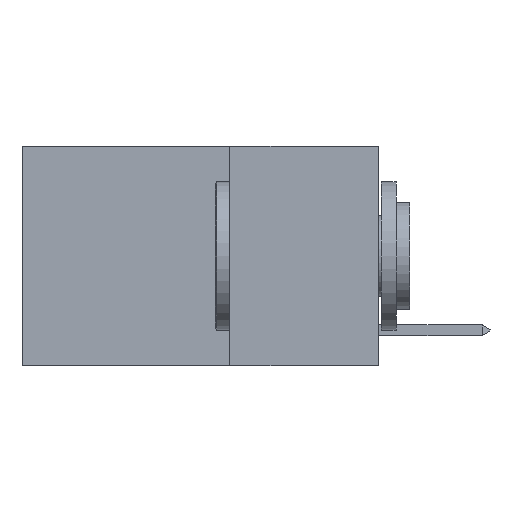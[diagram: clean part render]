
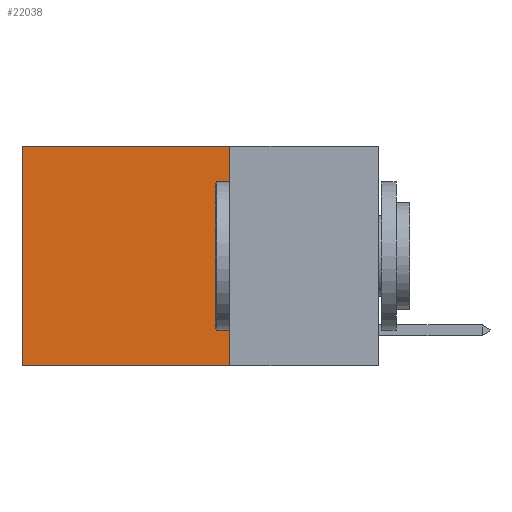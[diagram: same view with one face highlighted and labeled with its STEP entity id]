
A CAD part, left-side view. The second image highlights one B-rep face of the part: STEP entity #22038.
In plain terms, the highlighted planar face has unit normal (-1, 0, 0).
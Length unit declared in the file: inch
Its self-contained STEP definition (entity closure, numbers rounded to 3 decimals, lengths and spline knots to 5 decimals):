
#1754 = ORIENTED_EDGE ( 'NONE', *, *, #24520, .F. ) ;
#2118 = ORIENTED_EDGE ( 'NONE', *, *, #24918, .T. ) ;
#4122 = DIRECTION ( 'NONE',  ( 0., 1., 0. ) ) ;
#4167 = PLANE ( 'NONE',  #25455 ) ;
#5313 = VECTOR ( 'NONE', #19232, 39.37008 ) ;
#6423 = CARTESIAN_POINT ( 'NONE',  ( 0.2625, 0.25, 0. ) ) ;
#6466 = DIRECTION ( 'NONE',  ( 0., 0., -1. ) ) ;
#7605 = EDGE_CURVE ( 'NONE', #13305, #20000, #18055, .T. ) ;
#7867 = CARTESIAN_POINT ( 'NONE',  ( 0.2625, 0.25, -0.37 ) ) ;
#8535 = DIRECTION ( 'NONE',  ( 1., 0., 0. ) ) ;
#10118 = VECTOR ( 'NONE', #4122, 39.37008 ) ;
#10273 = CARTESIAN_POINT ( 'NONE',  ( 0.2625, 0.6, 0. ) ) ;
#10665 = FACE_OUTER_BOUND ( 'NONE', #19498, .T. ) ;
#11126 = ORIENTED_EDGE ( 'NONE', *, *, #19804, .T. ) ;
#12660 = LINE ( 'NONE', #25573, #5313 ) ;
#12701 = CARTESIAN_POINT ( 'NONE',  ( 0.2625, 0.25, 0. ) ) ;
#13259 = CARTESIAN_POINT ( 'NONE',  ( 0.2625, 0.25, 0. ) ) ;
#13305 = VERTEX_POINT ( 'NONE', #7867 ) ;
#14267 = CARTESIAN_POINT ( 'NONE',  ( 0.2625, 0.25, -0.37 ) ) ;
#14719 = ORIENTED_EDGE ( 'NONE', *, *, #7605, .F. ) ;
#14830 = CARTESIAN_POINT ( 'NONE',  ( 0.2625, 0.25, 0. ) ) ;
#15960 = DIRECTION ( 'NONE',  ( 0., 1., 0. ) ) ;
#17042 = LINE ( 'NONE', #12701, #10118 ) ;
#17125 = DIRECTION ( 'NONE',  ( 0., 0., -1. ) ) ;
#18055 = LINE ( 'NONE', #14267, #23469 ) ;
#19232 = DIRECTION ( 'NONE',  ( 0., 0., -1. ) ) ;
#19410 = VERTEX_POINT ( 'NONE', #14830 ) ;
#19498 = EDGE_LOOP ( 'NONE', ( #2118, #14719, #1754, #11126 ) ) ;
#19720 = VECTOR ( 'NONE', #6466, 39.37008 ) ;
#19804 = EDGE_CURVE ( 'NONE', #19410, #20028, #17042, .T. ) ;
#20000 = VERTEX_POINT ( 'NONE', #24901 ) ;
#20028 = VERTEX_POINT ( 'NONE', #10273 ) ;
#22038 = ADVANCED_FACE ( 'NONE', ( #10665 ), #4167, .F. ) ;
#23469 = VECTOR ( 'NONE', #15960, 39.37008 ) ;
#24520 = EDGE_CURVE ( 'NONE', #19410, #13305, #26014, .T. ) ;
#24901 = CARTESIAN_POINT ( 'NONE',  ( 0.2625, 0.6, -0.37 ) ) ;
#24918 = EDGE_CURVE ( 'NONE', #20028, #20000, #12660, .T. ) ;
#25455 = AXIS2_PLACEMENT_3D ( 'NONE', #6423, #8535, #17125 ) ;
#25573 = CARTESIAN_POINT ( 'NONE',  ( 0.2625, 0.6, 0. ) ) ;
#26014 = LINE ( 'NONE', #13259, #19720 ) ;
